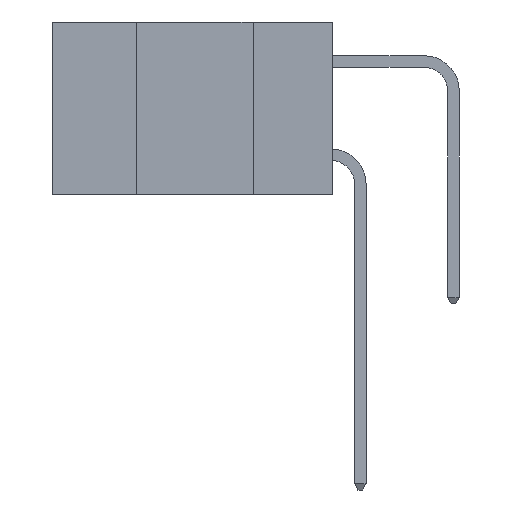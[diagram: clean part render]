
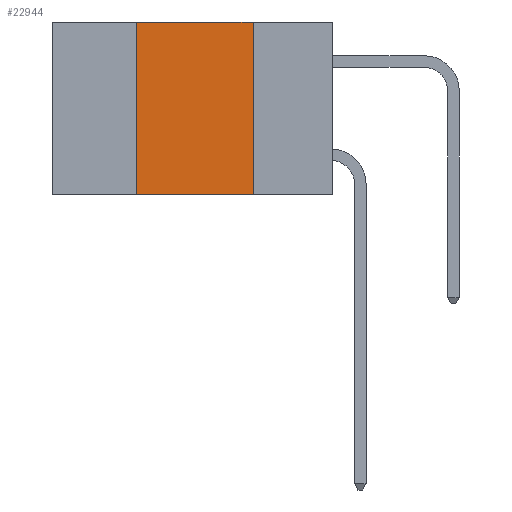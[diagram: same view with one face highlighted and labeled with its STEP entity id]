
A CAD part, left-side view. The second image highlights one B-rep face of the part: STEP entity #22944.
In plain terms, the highlighted planar face has unit normal (-1, 0, 0).
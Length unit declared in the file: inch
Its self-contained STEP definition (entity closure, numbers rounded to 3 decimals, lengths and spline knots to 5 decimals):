
#894 = CARTESIAN_POINT ( 'NONE',  ( 0., 0.42, 0. ) ) ;
#1486 = CARTESIAN_POINT ( 'NONE',  ( 0., 0.6, -0.37 ) ) ;
#2130 = DIRECTION ( 'NONE',  ( 0., -1., 0. ) ) ;
#2147 = CARTESIAN_POINT ( 'NONE',  ( 0., 0.17, -0.37 ) ) ;
#2561 = LINE ( 'NONE', #1486, #24932 ) ;
#2562 = VECTOR ( 'NONE', #8492, 39.37008 ) ;
#2878 = VERTEX_POINT ( 'NONE', #894 ) ;
#3777 = CARTESIAN_POINT ( 'NONE',  ( 0., 0.17, 0. ) ) ;
#6818 = EDGE_CURVE ( 'NONE', #17852, #12118, #19918, .T. ) ;
#8492 = DIRECTION ( 'NONE',  ( 0., 0., -1. ) ) ;
#11180 = LINE ( 'NONE', #25684, #22680 ) ;
#11295 = CARTESIAN_POINT ( 'NONE',  ( 0., 0.6, 0. ) ) ;
#12118 = VERTEX_POINT ( 'NONE', #2147 ) ;
#12651 = ORIENTED_EDGE ( 'NONE', *, *, #14970, .F. ) ;
#12827 = DIRECTION ( 'NONE',  ( 0., 0., 1. ) ) ;
#13256 = EDGE_LOOP ( 'NONE', ( #22777, #23434, #12651, #24763 ) ) ;
#13506 = DIRECTION ( 'NONE',  ( 0., 0., -1. ) ) ;
#14502 = VERTEX_POINT ( 'NONE', #22018 ) ;
#14970 = EDGE_CURVE ( 'NONE', #14502, #2878, #11180, .T. ) ;
#15215 = CARTESIAN_POINT ( 'NONE',  ( 0., 0.6, 0. ) ) ;
#15369 = VECTOR ( 'NONE', #2130, 39.37008 ) ;
#16230 = FACE_OUTER_BOUND ( 'NONE', #13256, .T. ) ;
#16761 = CARTESIAN_POINT ( 'NONE',  ( 0., 0.17, -0.37 ) ) ;
#17852 = VERTEX_POINT ( 'NONE', #3777 ) ;
#19037 = DIRECTION ( 'NONE',  ( 0., -1., 0. ) ) ;
#19918 = LINE ( 'NONE', #16761, #2562 ) ;
#20063 = EDGE_CURVE ( 'NONE', #2878, #17852, #26094, .T. ) ;
#22018 = CARTESIAN_POINT ( 'NONE',  ( 0., 0.42, -0.37 ) ) ;
#22680 = VECTOR ( 'NONE', #12827, 39.37008 ) ;
#22777 = ORIENTED_EDGE ( 'NONE', *, *, #6818, .F. ) ;
#22944 = ADVANCED_FACE ( 'NONE', ( #16230 ), #24213, .F. ) ;
#23434 = ORIENTED_EDGE ( 'NONE', *, *, #20063, .F. ) ;
#24213 = PLANE ( 'NONE',  #25483 ) ;
#24763 = ORIENTED_EDGE ( 'NONE', *, *, #28087, .T. ) ;
#24932 = VECTOR ( 'NONE', #19037, 39.37008 ) ;
#25483 = AXIS2_PLACEMENT_3D ( 'NONE', #11295, #26343, #13506 ) ;
#25684 = CARTESIAN_POINT ( 'NONE',  ( 0., 0.42, -0.37 ) ) ;
#26094 = LINE ( 'NONE', #15215, #15369 ) ;
#26343 = DIRECTION ( 'NONE',  ( 1., 0., 0. ) ) ;
#28087 = EDGE_CURVE ( 'NONE', #14502, #12118, #2561, .T. ) ;
